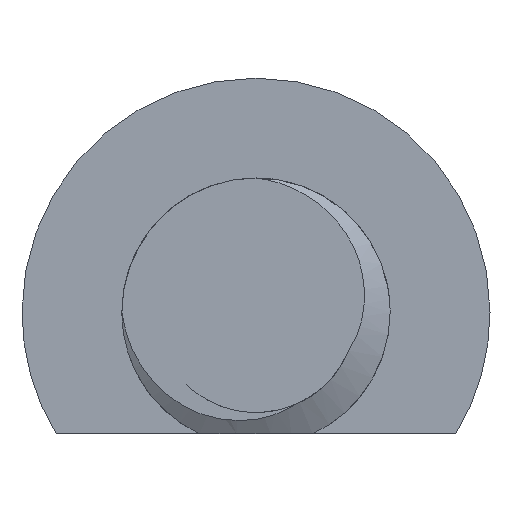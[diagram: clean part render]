
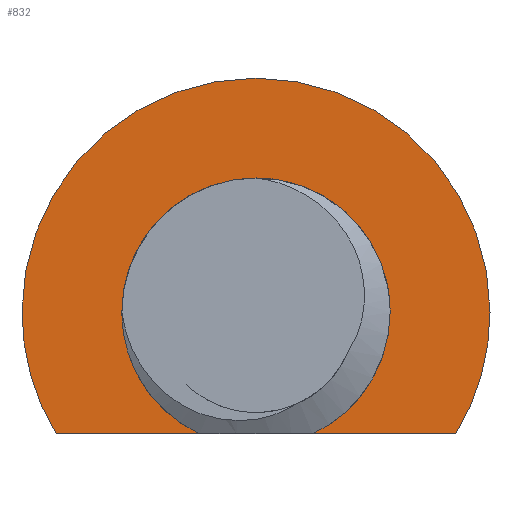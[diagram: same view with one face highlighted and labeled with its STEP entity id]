
A CAD part, left-side view. The second image highlights one B-rep face of the part: STEP entity #832.
In plain terms, the highlighted planar face has unit normal (-1, 0, 0).
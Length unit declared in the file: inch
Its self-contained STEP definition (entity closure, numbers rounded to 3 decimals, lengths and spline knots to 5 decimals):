
#89 = CARTESIAN_POINT ( 'NONE',  ( 1.22162, 0.245, 1.11338 ) ) ;
#99 = DIRECTION ( 'NONE',  ( 1., 0., 0. ) ) ;
#134 = DIRECTION ( 'NONE',  ( 0., 1., 0. ) ) ;
#146 = DIRECTION ( 'NONE',  ( 0., 1., 0. ) ) ;
#176 = CARTESIAN_POINT ( 'NONE',  ( 1.22162, 0.1375, 1.11338 ) ) ;
#243 = AXIS2_PLACEMENT_3D ( 'NONE', #551, #1043, #2263 ) ;
#281 = VERTEX_POINT ( 'NONE', #1542 ) ;
#335 = CARTESIAN_POINT ( 'NONE',  ( 1.22162, 0.1375, 1.11338 ) ) ;
#405 = DIRECTION ( 'NONE',  ( 0., 1., 0. ) ) ;
#466 = VERTEX_POINT ( 'NONE', #1854 ) ;
#470 = ORIENTED_EDGE ( 'NONE', *, *, #2394, .F. ) ;
#477 = VECTOR ( 'NONE', #2349, 39.37008 ) ;
#495 = CIRCLE ( 'NONE', #911, 0.1075 ) ;
#551 = CARTESIAN_POINT ( 'NONE',  ( 1.22162, 0.1375, 1.11338 ) ) ;
#603 = EDGE_CURVE ( 'NONE', #1422, #2463, #1972, .T. ) ;
#671 = ORIENTED_EDGE ( 'NONE', *, *, #757, .F. ) ;
#725 = ORIENTED_EDGE ( 'NONE', *, *, #1793, .T. ) ;
#745 = VERTEX_POINT ( 'NONE', #1831 ) ;
#757 = EDGE_CURVE ( 'NONE', #2334, #466, #2362, .T. ) ;
#815 = EDGE_CURVE ( 'NONE', #281, #1820, #2626, .T. ) ;
#832 = ADVANCED_FACE ( 'NONE', ( #2735 ), #1595, .F. ) ;
#838 = DIRECTION ( 'NONE',  ( 0., 1., 0. ) ) ;
#862 = ORIENTED_EDGE ( 'NONE', *, *, #2659, .F. ) ;
#911 = AXIS2_PLACEMENT_3D ( 'NONE', #1078, #99, #838 ) ;
#1032 = AXIS2_PLACEMENT_3D ( 'NONE', #335, #1081, #134 ) ;
#1043 = DIRECTION ( 'NONE',  ( 1., 0., 0. ) ) ;
#1078 = CARTESIAN_POINT ( 'NONE',  ( 1.22162, 0.1375, 1.11338 ) ) ;
#1081 = DIRECTION ( 'NONE',  ( 1., 0., 0. ) ) ;
#1122 = ORIENTED_EDGE ( 'NONE', *, *, #2144, .T. ) ;
#1214 = AXIS2_PLACEMENT_3D ( 'NONE', #1327, #2542, #2034 ) ;
#1236 = CARTESIAN_POINT ( 'NONE',  ( 1.22162, -0.02266, 1.01588 ) ) ;
#1282 = ORIENTED_EDGE ( 'NONE', *, *, #2921, .T. ) ;
#1327 = CARTESIAN_POINT ( 'NONE',  ( 1.22162, 0.1375, 1.11338 ) ) ;
#1373 = CARTESIAN_POINT ( 'NONE',  ( 1.22162, 0.03, 1.11338 ) ) ;
#1422 = VERTEX_POINT ( 'NONE', #1891 ) ;
#1464 = VERTEX_POINT ( 'NONE', #1373 ) ;
#1476 = LINE ( 'NONE', #3093, #1517 ) ;
#1517 = VECTOR ( 'NONE', #1657, 39.37008 ) ;
#1542 = CARTESIAN_POINT ( 'NONE',  ( 1.22162, 0.18278, 1.01588 ) ) ;
#1595 = PLANE ( 'NONE',  #1757 ) ;
#1657 = DIRECTION ( 'NONE',  ( 0., -1., 0. ) ) ;
#1712 = DIRECTION ( 'NONE',  ( 0., 1., 0. ) ) ;
#1757 = AXIS2_PLACEMENT_3D ( 'NONE', #176, #3044, #146 ) ;
#1793 = EDGE_CURVE ( 'NONE', #1464, #1422, #2429, .T. ) ;
#1820 = VERTEX_POINT ( 'NONE', #89 ) ;
#1831 = CARTESIAN_POINT ( 'NONE',  ( 1.22162, -0.05, 1.11338 ) ) ;
#1854 = CARTESIAN_POINT ( 'NONE',  ( 1.22162, 0.325, 1.11338 ) ) ;
#1861 = DIRECTION ( 'NONE',  ( 1., 0., 0. ) ) ;
#1891 = CARTESIAN_POINT ( 'NONE',  ( 1.22162, 0.09222, 1.01588 ) ) ;
#1924 = DIRECTION ( 'NONE',  ( 1., 0., 0. ) ) ;
#1972 = LINE ( 'NONE', #3051, #477 ) ;
#2034 = DIRECTION ( 'NONE',  ( 0., 1., 0. ) ) ;
#2138 = EDGE_LOOP ( 'NONE', ( #671, #1122, #2392, #1282, #725, #3027, #470, #862 ) ) ;
#2144 = EDGE_CURVE ( 'NONE', #2334, #281, #1476, .T. ) ;
#2263 = DIRECTION ( 'NONE',  ( 0., 1., 0. ) ) ;
#2334 = VERTEX_POINT ( 'NONE', #2888 ) ;
#2349 = DIRECTION ( 'NONE',  ( 0., -1., 0. ) ) ;
#2362 = CIRCLE ( 'NONE', #1032, 0.1875 ) ;
#2392 = ORIENTED_EDGE ( 'NONE', *, *, #815, .T. ) ;
#2394 = EDGE_CURVE ( 'NONE', #745, #2463, #2530, .T. ) ;
#2429 = CIRCLE ( 'NONE', #1214, 0.1075 ) ;
#2438 = CIRCLE ( 'NONE', #243, 0.1875 ) ;
#2452 = AXIS2_PLACEMENT_3D ( 'NONE', #2824, #1861, #405 ) ;
#2463 = VERTEX_POINT ( 'NONE', #1236 ) ;
#2530 = CIRCLE ( 'NONE', #3100, 0.1875 ) ;
#2542 = DIRECTION ( 'NONE',  ( 1., 0., 0. ) ) ;
#2626 = CIRCLE ( 'NONE', #2452, 0.1075 ) ;
#2659 = EDGE_CURVE ( 'NONE', #466, #745, #2438, .T. ) ;
#2735 = FACE_OUTER_BOUND ( 'NONE', #2138, .T. ) ;
#2824 = CARTESIAN_POINT ( 'NONE',  ( 1.22162, 0.1375, 1.11338 ) ) ;
#2888 = CARTESIAN_POINT ( 'NONE',  ( 1.22162, 0.29766, 1.01588 ) ) ;
#2904 = CARTESIAN_POINT ( 'NONE',  ( 1.22162, 0.1375, 1.11338 ) ) ;
#2921 = EDGE_CURVE ( 'NONE', #1820, #1464, #495, .T. ) ;
#3027 = ORIENTED_EDGE ( 'NONE', *, *, #603, .T. ) ;
#3044 = DIRECTION ( 'NONE',  ( 1., 0., 0. ) ) ;
#3051 = CARTESIAN_POINT ( 'NONE',  ( 1.22162, 0.1375, 1.01588 ) ) ;
#3093 = CARTESIAN_POINT ( 'NONE',  ( 1.22162, 0.1375, 1.01588 ) ) ;
#3100 = AXIS2_PLACEMENT_3D ( 'NONE', #2904, #1924, #1712 ) ;
